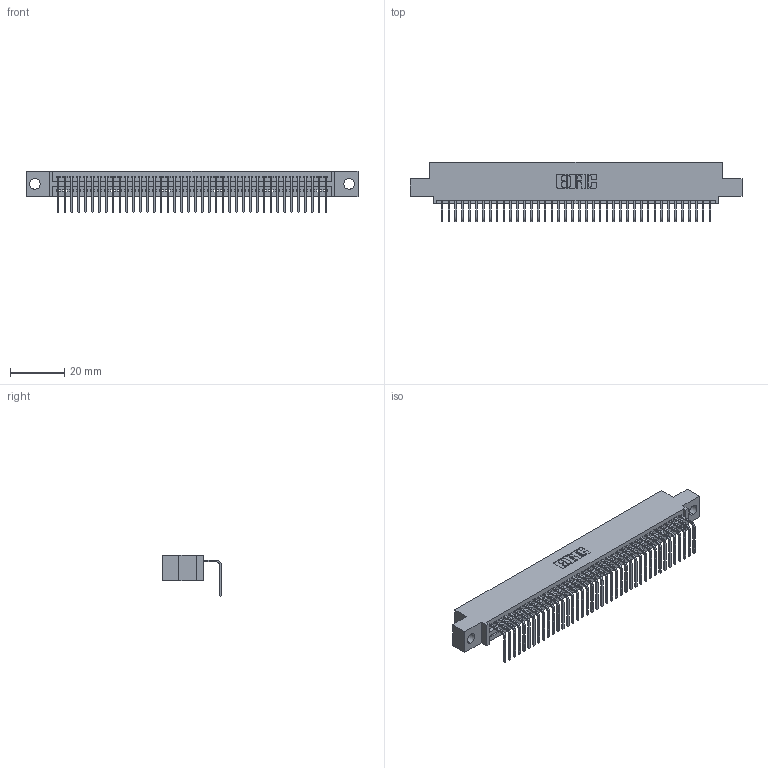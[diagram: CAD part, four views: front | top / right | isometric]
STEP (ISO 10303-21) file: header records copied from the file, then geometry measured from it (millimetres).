
FILE_DESCRIPTION (( 'STEP AP203' ), '1' );
FILE_NAME ('345-040-558-404.STEP', '2021-06-09T16:42:57', ( '' ), ( '' ), 'SwSTEP 2.0', 'SolidWorks 2020', '' );
FILE_SCHEMA (( 'CONFIG_CONTROL_DESIGN' ));
Length unit declared in the file: inch
Products named in the file (3): 345-292-001_558 Tail - 2; 345-040-558-404; 345 Part_0.110 Offset - 0.156 Dia-TI
Assembly tree (41 placements, depth 2):
  345-040-558-404
    345 Part_0.110 Offset - 0.156 Dia-TI
    345-292-001_558 Tail - 2  x40
Bounding box: 122.81 x 21.83 x 15.37 mm (x, y, z)
Volume: 11602.1 mm3; surface area: 16098.4 mm2
Topology: 41 solids, 41 shells, 2544 faces, 7669 edges, 5058 vertices
Faces by surface type: plane 1778, cylinder 766
Entity records: 31009 total; most frequent: CARTESIAN_POINT 5382, ORIENTED_EDGE 5354, DIRECTION 4701, EDGE_CURVE 2677, VECTOR 2385, LINE 2385, VERTEX_POINT 1782, AXIS2_PLACEMENT_3D 1158
